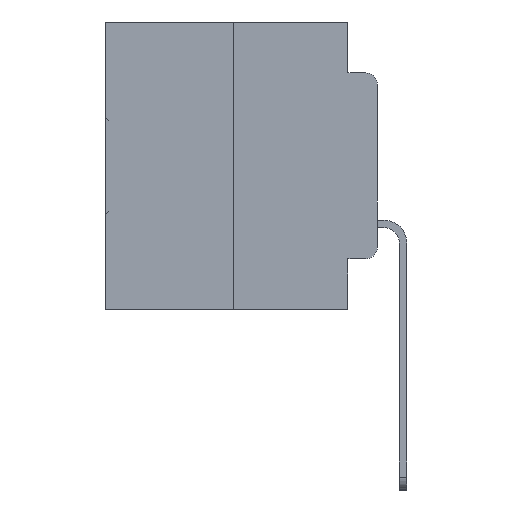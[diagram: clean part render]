
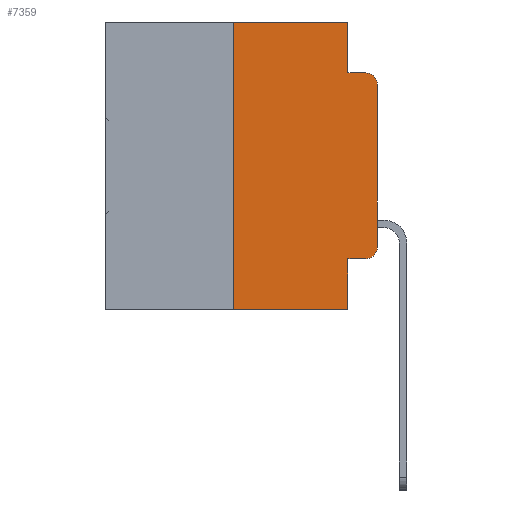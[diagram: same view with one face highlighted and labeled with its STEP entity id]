
A CAD part, left-side view. The second image highlights one B-rep face of the part: STEP entity #7359.
In plain terms, the highlighted planar face has unit normal (-1, 0, 0).
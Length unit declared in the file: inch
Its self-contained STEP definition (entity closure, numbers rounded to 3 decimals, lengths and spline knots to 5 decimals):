
#151 = ORIENTED_EDGE ( 'NONE', *, *, #25489, .F. ) ;
#865 = VECTOR ( 'NONE', #6201, 39.37008 ) ;
#956 = VECTOR ( 'NONE', #30557, 39.37008 ) ;
#1871 = VECTOR ( 'NONE', #22367, 39.37008 ) ;
#2025 = CARTESIAN_POINT ( 'NONE',  ( 0., 0.051, -0.5 ) ) ;
#2134 = CARTESIAN_POINT ( 'NONE',  ( 0., 0.02, -0.1085 ) ) ;
#2654 = ORIENTED_EDGE ( 'NONE', *, *, #22365, .F. ) ;
#2968 = FACE_OUTER_BOUND ( 'NONE', #16026, .T. ) ;
#3315 = CARTESIAN_POINT ( 'NONE',  ( 0., 0.02, -0.3915 ) ) ;
#3606 = CARTESIAN_POINT ( 'NONE',  ( 0., 0.051, 0. ) ) ;
#3628 = EDGE_CURVE ( 'NONE', #5938, #8200, #5959, .T. ) ;
#3949 = VERTEX_POINT ( 'NONE', #23713 ) ;
#4622 = CARTESIAN_POINT ( 'NONE',  ( 0., 0., -0.1085 ) ) ;
#4742 = DIRECTION ( 'NONE',  ( 0., 0., -1. ) ) ;
#5170 = VECTOR ( 'NONE', #7716, 39.37008 ) ;
#5911 = DIRECTION ( 'NONE',  ( 0., 0., -1. ) ) ;
#5938 = VERTEX_POINT ( 'NONE', #30669 ) ;
#5959 = LINE ( 'NONE', #24569, #5170 ) ;
#6050 = EDGE_CURVE ( 'NONE', #24922, #13080, #29230, .T. ) ;
#6130 = CARTESIAN_POINT ( 'NONE',  ( 0., 0.473, -0.5 ) ) ;
#6201 = DIRECTION ( 'NONE',  ( 0., 0., -1. ) ) ;
#6612 = DIRECTION ( 'NONE',  ( 1., 0., 0. ) ) ;
#7359 = ADVANCED_FACE ( 'NONE', ( #2968 ), #16464, .F. ) ;
#7716 = DIRECTION ( 'NONE',  ( 0., 0., 1. ) ) ;
#7855 = LINE ( 'NONE', #9114, #956 ) ;
#8103 = LINE ( 'NONE', #26206, #26490 ) ;
#8200 = VERTEX_POINT ( 'NONE', #4622 ) ;
#8759 = VERTEX_POINT ( 'NONE', #19604 ) ;
#9114 = CARTESIAN_POINT ( 'NONE',  ( 0., 0.25, 0. ) ) ;
#9323 = CARTESIAN_POINT ( 'NONE',  ( 0., 0.25, -0.5 ) ) ;
#9425 = ORIENTED_EDGE ( 'NONE', *, *, #22179, .T. ) ;
#11074 = ORIENTED_EDGE ( 'NONE', *, *, #19205, .T. ) ;
#11607 = CARTESIAN_POINT ( 'NONE',  ( 0., 0.473, 0. ) ) ;
#12635 = ORIENTED_EDGE ( 'NONE', *, *, #12796, .T. ) ;
#12796 = EDGE_CURVE ( 'NONE', #25708, #5938, #24457, .T. ) ;
#12985 = ORIENTED_EDGE ( 'NONE', *, *, #3628, .T. ) ;
#13080 = VERTEX_POINT ( 'NONE', #24151 ) ;
#15127 = LINE ( 'NONE', #3606, #865 ) ;
#15304 = LINE ( 'NONE', #29267, #1871 ) ;
#16026 = EDGE_LOOP ( 'NONE', ( #12985, #19349, #151, #27033, #21541, #2654, #9425, #23030, #11074, #12635 ) ) ;
#16144 = CIRCLE ( 'NONE', #29687, 0.02 ) ;
#16464 = PLANE ( 'NONE',  #29260 ) ;
#16976 = CARTESIAN_POINT ( 'NONE',  ( 0., 0.25, 0. ) ) ;
#17027 = VERTEX_POINT ( 'NONE', #27533 ) ;
#18116 = AXIS2_PLACEMENT_3D ( 'NONE', #3315, #20604, #5911 ) ;
#19205 = EDGE_CURVE ( 'NONE', #8759, #25708, #27055, .T. ) ;
#19349 = ORIENTED_EDGE ( 'NONE', *, *, #28579, .T. ) ;
#19536 = DIRECTION ( 'NONE',  ( -1., 0., 0. ) ) ;
#19604 = CARTESIAN_POINT ( 'NONE',  ( 0., 0.051, -0.4115 ) ) ;
#19701 = LINE ( 'NONE', #6130, #31350 ) ;
#19763 = VERTEX_POINT ( 'NONE', #2025 ) ;
#20117 = VECTOR ( 'NONE', #27658, 39.37008 ) ;
#20604 = DIRECTION ( 'NONE',  ( -1., 0., 0. ) ) ;
#20778 = EDGE_CURVE ( 'NONE', #8759, #19763, #15304, .T. ) ;
#21497 = DIRECTION ( 'NONE',  ( 0., -1., 0. ) ) ;
#21541 = ORIENTED_EDGE ( 'NONE', *, *, #6050, .F. ) ;
#21605 = DIRECTION ( 'NONE',  ( 0., -1., 0. ) ) ;
#22179 = EDGE_CURVE ( 'NONE', #22445, #19763, #19701, .T. ) ;
#22331 = VECTOR ( 'NONE', #21605, 39.37008 ) ;
#22365 = EDGE_CURVE ( 'NONE', #22445, #24922, #7855, .T. ) ;
#22367 = DIRECTION ( 'NONE',  ( 0., 0., -1. ) ) ;
#22445 = VERTEX_POINT ( 'NONE', #9323 ) ;
#23030 = ORIENTED_EDGE ( 'NONE', *, *, #20778, .F. ) ;
#23573 = DIRECTION ( 'NONE',  ( 0., 0., -1. ) ) ;
#23713 = CARTESIAN_POINT ( 'NONE',  ( 0., 0.051, -0.0885 ) ) ;
#23916 = EDGE_CURVE ( 'NONE', #13080, #3949, #15127, .T. ) ;
#23963 = CARTESIAN_POINT ( 'NONE',  ( 0., 0.473, 0. ) ) ;
#24151 = CARTESIAN_POINT ( 'NONE',  ( 0., 0.051, 0. ) ) ;
#24457 = CIRCLE ( 'NONE', #18116, 0.02 ) ;
#24569 = CARTESIAN_POINT ( 'NONE',  ( 0., 0., 0. ) ) ;
#24922 = VERTEX_POINT ( 'NONE', #16976 ) ;
#25309 = CARTESIAN_POINT ( 'NONE',  ( 0., 0.051, -0.4115 ) ) ;
#25489 = EDGE_CURVE ( 'NONE', #3949, #17027, #8103, .T. ) ;
#25501 = DIRECTION ( 'NONE',  ( 0., -1., 0. ) ) ;
#25708 = VERTEX_POINT ( 'NONE', #31476 ) ;
#26206 = CARTESIAN_POINT ( 'NONE',  ( 0., 0.051, -0.0885 ) ) ;
#26490 = VECTOR ( 'NONE', #21497, 39.37008 ) ;
#27033 = ORIENTED_EDGE ( 'NONE', *, *, #23916, .F. ) ;
#27055 = LINE ( 'NONE', #25309, #20117 ) ;
#27533 = CARTESIAN_POINT ( 'NONE',  ( 0., 0.02, -0.0885 ) ) ;
#27658 = DIRECTION ( 'NONE',  ( 0., -1., 0. ) ) ;
#28579 = EDGE_CURVE ( 'NONE', #8200, #17027, #16144, .T. ) ;
#29230 = LINE ( 'NONE', #23963, #22331 ) ;
#29260 = AXIS2_PLACEMENT_3D ( 'NONE', #11607, #6612, #23573 ) ;
#29267 = CARTESIAN_POINT ( 'NONE',  ( 0., 0.051, 0. ) ) ;
#29687 = AXIS2_PLACEMENT_3D ( 'NONE', #2134, #19536, #4742 ) ;
#30557 = DIRECTION ( 'NONE',  ( 0., 0., 1. ) ) ;
#30669 = CARTESIAN_POINT ( 'NONE',  ( 0., 0., -0.3915 ) ) ;
#31350 = VECTOR ( 'NONE', #25501, 39.37008 ) ;
#31476 = CARTESIAN_POINT ( 'NONE',  ( 0., 0.02, -0.4115 ) ) ;
